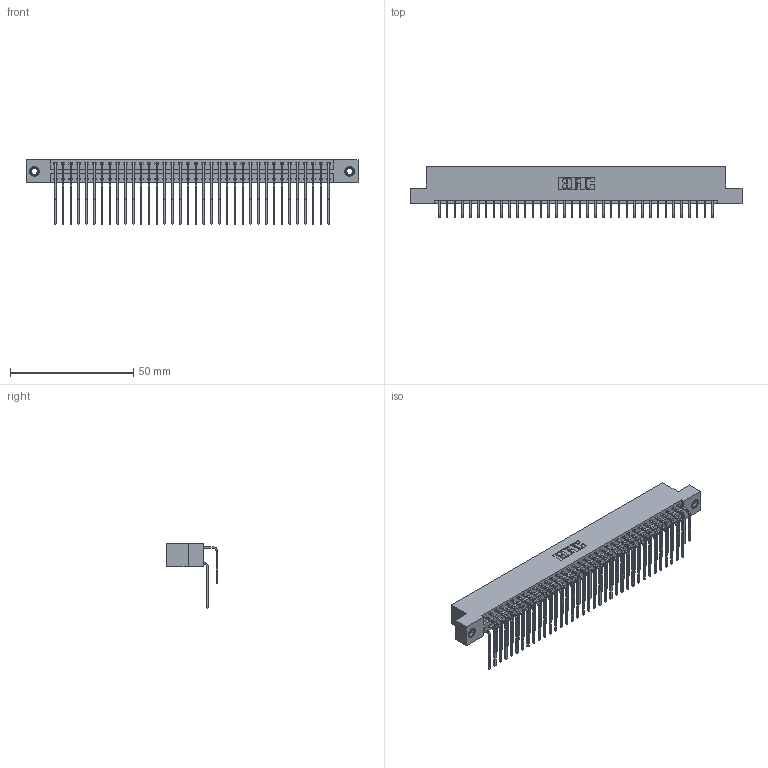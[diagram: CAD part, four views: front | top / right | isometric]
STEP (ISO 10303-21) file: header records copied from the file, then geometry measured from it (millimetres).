
FILE_DESCRIPTION (( 'STEP AP203' ), '1' );
FILE_NAME ('396-072-559-207.STEP', '2018-09-09T10:57:46', ( '' ), ( '' ), 'SwSTEP 2.0', 'SolidWorks 2016', '' );
FILE_SCHEMA (( 'CONFIG_CONTROL_DESIGN' ));
Length unit declared in the file: inch
Products named in the file (5): 396-072-559-207; 346 Part_Flush Mounting Lugs - 0.156 Dia-TI; 345-292-001_558 559 Tail - 1; 345-292-001_559 Tail - 2; 345-250-001_345-250-005-103
Assembly tree (75 placements, depth 2):
  396-072-559-207
    346 Part_Flush Mounting Lugs - 0.156 Dia-TI
    345-292-001_558 559 Tail - 1  x36
    345-292-001_559 Tail - 2  x36
    345-250-001_345-250-005-103  x2
Bounding box: 134.87 x 20.89 x 26.16 mm (x, y, z)
Volume: 13507.1 mm3; surface area: 20498.5 mm2
Topology: 75 solids, 75 shells, 4070 faces, 12057 edges, 7934 vertices
Faces by surface type: plane 2772, cylinder 1282, cone 12, torus 4
Entity records: 27272 total; most frequent: CARTESIAN_POINT 4538, ORIENTED_EDGE 4414, DIRECTION 4049, EDGE_CURVE 2207, LINE 1871, VECTOR 1871, VERTEX_POINT 1464, AXIS2_PLACEMENT_3D 1089
